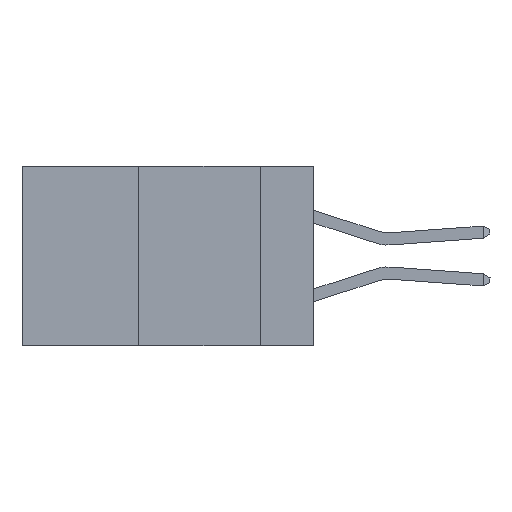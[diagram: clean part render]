
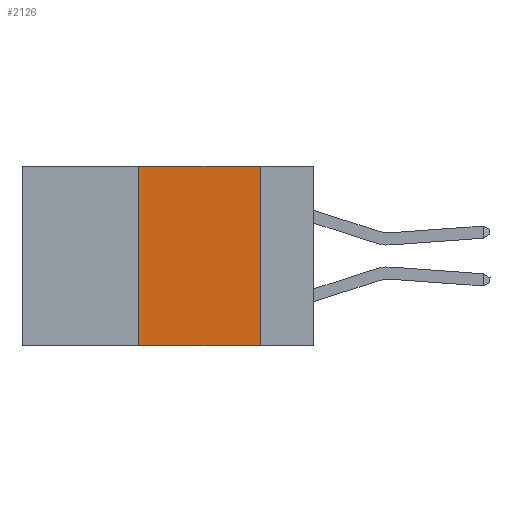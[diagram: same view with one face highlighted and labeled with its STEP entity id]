
A CAD part, left-side view. The second image highlights one B-rep face of the part: STEP entity #2126.
In plain terms, the highlighted planar face has unit normal (-1, 0, 0).
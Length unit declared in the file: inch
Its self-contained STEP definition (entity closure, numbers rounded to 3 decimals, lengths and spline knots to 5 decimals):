
#387 = DIRECTION ( 'NONE',  ( 0., 0., -1. ) ) ;
#1212 = LINE ( 'NONE', #4822, #8873 ) ;
#1262 = LINE ( 'NONE', #5457, #5970 ) ;
#1286 = DIRECTION ( 'NONE',  ( 1., 0., 0. ) ) ;
#1371 = VERTEX_POINT ( 'NONE', #6578 ) ;
#2116 = CARTESIAN_POINT ( 'NONE',  ( 0., 0.36, -0.37 ) ) ;
#2126 = ADVANCED_FACE ( 'NONE', ( #3793 ), #7305, .F. ) ;
#2601 = EDGE_CURVE ( 'NONE', #1371, #11174, #3937, .T. ) ;
#3112 = CARTESIAN_POINT ( 'NONE',  ( 0., 0.6, -0.37 ) ) ;
#3138 = EDGE_LOOP ( 'NONE', ( #7743, #10201, #7334, #5866 ) ) ;
#3793 = FACE_OUTER_BOUND ( 'NONE', #3138, .T. ) ;
#3937 = LINE ( 'NONE', #4079, #6447 ) ;
#4079 = CARTESIAN_POINT ( 'NONE',  ( 0., 0.6, 0. ) ) ;
#4822 = CARTESIAN_POINT ( 'NONE',  ( 0., 0.11, 0. ) ) ;
#5189 = DIRECTION ( 'NONE',  ( 0., -1., 0. ) ) ;
#5457 = CARTESIAN_POINT ( 'NONE',  ( 0., 0.36, 0. ) ) ;
#5866 = ORIENTED_EDGE ( 'NONE', *, *, #12285, .T. ) ;
#5970 = VECTOR ( 'NONE', #7353, 39.37008 ) ;
#5986 = VECTOR ( 'NONE', #5189, 39.37008 ) ;
#6192 = AXIS2_PLACEMENT_3D ( 'NONE', #11433, #1286, #387 ) ;
#6447 = VECTOR ( 'NONE', #7062, 39.37008 ) ;
#6578 = CARTESIAN_POINT ( 'NONE',  ( 0., 0.36, 0. ) ) ;
#7062 = DIRECTION ( 'NONE',  ( 0., -1., 0. ) ) ;
#7305 = PLANE ( 'NONE',  #6192 ) ;
#7334 = ORIENTED_EDGE ( 'NONE', *, *, #12958, .F. ) ;
#7353 = DIRECTION ( 'NONE',  ( 0., 0., 1. ) ) ;
#7700 = LINE ( 'NONE', #3112, #5986 ) ;
#7743 = ORIENTED_EDGE ( 'NONE', *, *, #9774, .F. ) ;
#8655 = VERTEX_POINT ( 'NONE', #2116 ) ;
#8873 = VECTOR ( 'NONE', #11804, 39.37008 ) ;
#9774 = EDGE_CURVE ( 'NONE', #11174, #12952, #1212, .T. ) ;
#10201 = ORIENTED_EDGE ( 'NONE', *, *, #2601, .F. ) ;
#10492 = CARTESIAN_POINT ( 'NONE',  ( 0., 0.11, 0. ) ) ;
#11174 = VERTEX_POINT ( 'NONE', #10492 ) ;
#11433 = CARTESIAN_POINT ( 'NONE',  ( 0., 0.6, 0. ) ) ;
#11804 = DIRECTION ( 'NONE',  ( 0., 0., -1. ) ) ;
#12285 = EDGE_CURVE ( 'NONE', #8655, #12952, #7700, .T. ) ;
#12436 = CARTESIAN_POINT ( 'NONE',  ( 0., 0.11, -0.37 ) ) ;
#12952 = VERTEX_POINT ( 'NONE', #12436 ) ;
#12958 = EDGE_CURVE ( 'NONE', #8655, #1371, #1262, .T. ) ;
